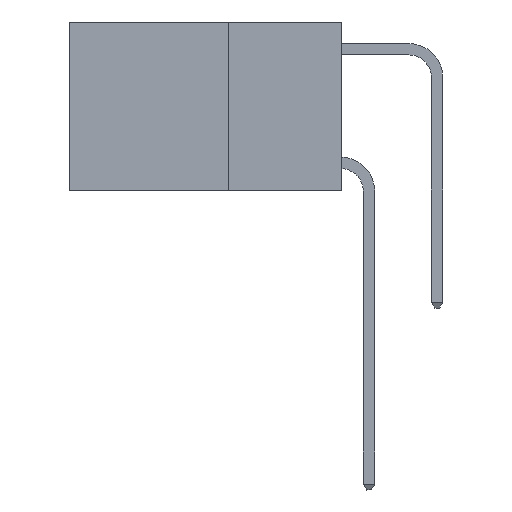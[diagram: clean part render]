
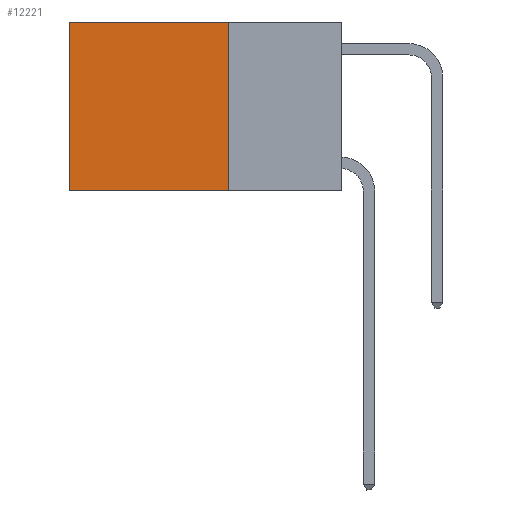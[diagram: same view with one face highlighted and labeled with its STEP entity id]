
A CAD part, left-side view. The second image highlights one B-rep face of the part: STEP entity #12221.
In plain terms, the highlighted planar face has unit normal (-1, 0, 0).
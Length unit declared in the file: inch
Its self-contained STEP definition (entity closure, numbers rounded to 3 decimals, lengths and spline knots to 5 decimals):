
#261 = ORIENTED_EDGE ( 'NONE', *, *, #897, .F. ) ;
#404 = EDGE_CURVE ( 'NONE', #16162, #11296, #8607, .T. ) ;
#897 = EDGE_CURVE ( 'NONE', #6203, #10058, #16178, .T. ) ;
#1393 = VECTOR ( 'NONE', #5916, 39.37008 ) ;
#2513 = ORIENTED_EDGE ( 'NONE', *, *, #14819, .T. ) ;
#3034 = CARTESIAN_POINT ( 'NONE',  ( 0.2625, 0.25, -0.37 ) ) ;
#3072 = ORIENTED_EDGE ( 'NONE', *, *, #15727, .F. ) ;
#3976 = DIRECTION ( 'NONE',  ( 0., 0., -1. ) ) ;
#5114 = DIRECTION ( 'NONE',  ( 1., 0., 0. ) ) ;
#5906 = CARTESIAN_POINT ( 'NONE',  ( 0.2625, 0.25, 0. ) ) ;
#5916 = DIRECTION ( 'NONE',  ( 0., 1., 0. ) ) ;
#6203 = VERTEX_POINT ( 'NONE', #9322 ) ;
#7301 = DIRECTION ( 'NONE',  ( 0., 1., 0. ) ) ;
#7876 = CARTESIAN_POINT ( 'NONE',  ( 0.2625, 0.6, 0. ) ) ;
#8095 = AXIS2_PLACEMENT_3D ( 'NONE', #9292, #5114, #3976 ) ;
#8607 = LINE ( 'NONE', #13908, #14313 ) ;
#9039 = VECTOR ( 'NONE', #14000, 39.37008 ) ;
#9292 = CARTESIAN_POINT ( 'NONE',  ( 0.2625, 0.25, 0. ) ) ;
#9322 = CARTESIAN_POINT ( 'NONE',  ( 0.2625, 0.25, -0.37 ) ) ;
#10058 = VERTEX_POINT ( 'NONE', #12068 ) ;
#10195 = LINE ( 'NONE', #5906, #9039 ) ;
#10680 = VECTOR ( 'NONE', #15900, 39.37008 ) ;
#11296 = VERTEX_POINT ( 'NONE', #7876 ) ;
#11720 = FACE_OUTER_BOUND ( 'NONE', #14869, .T. ) ;
#12068 = CARTESIAN_POINT ( 'NONE',  ( 0.2625, 0.6, -0.37 ) ) ;
#12221 = ADVANCED_FACE ( 'NONE', ( #11720 ), #17028, .F. ) ;
#13125 = ORIENTED_EDGE ( 'NONE', *, *, #404, .T. ) ;
#13209 = LINE ( 'NONE', #14748, #10680 ) ;
#13908 = CARTESIAN_POINT ( 'NONE',  ( 0.2625, 0.25, 0. ) ) ;
#14000 = DIRECTION ( 'NONE',  ( 0., 0., -1. ) ) ;
#14313 = VECTOR ( 'NONE', #7301, 39.37008 ) ;
#14748 = CARTESIAN_POINT ( 'NONE',  ( 0.2625, 0.6, 0. ) ) ;
#14819 = EDGE_CURVE ( 'NONE', #11296, #10058, #13209, .T. ) ;
#14869 = EDGE_LOOP ( 'NONE', ( #2513, #261, #3072, #13125 ) ) ;
#15727 = EDGE_CURVE ( 'NONE', #16162, #6203, #10195, .T. ) ;
#15900 = DIRECTION ( 'NONE',  ( 0., 0., -1. ) ) ;
#16162 = VERTEX_POINT ( 'NONE', #16209 ) ;
#16178 = LINE ( 'NONE', #3034, #1393 ) ;
#16209 = CARTESIAN_POINT ( 'NONE',  ( 0.2625, 0.25, 0. ) ) ;
#17028 = PLANE ( 'NONE',  #8095 ) ;
